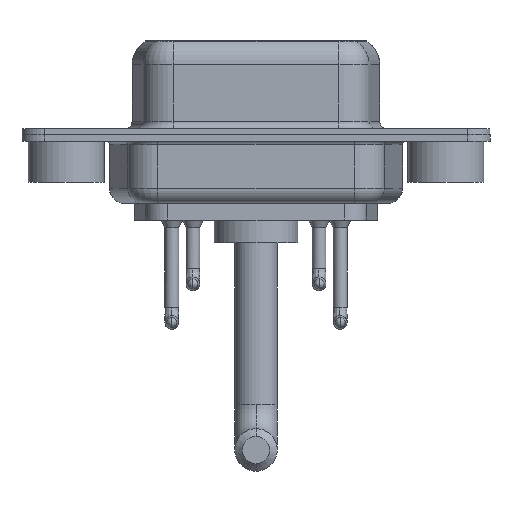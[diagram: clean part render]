
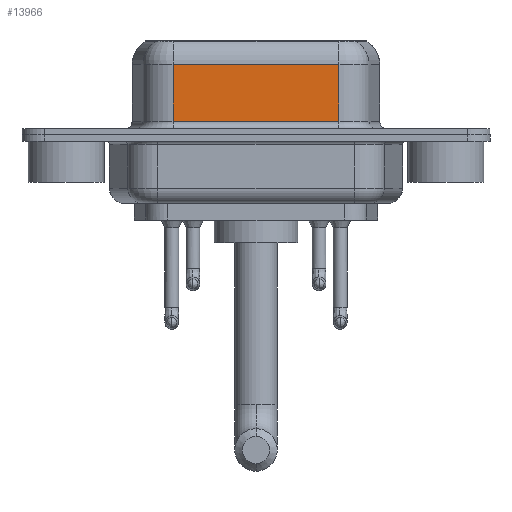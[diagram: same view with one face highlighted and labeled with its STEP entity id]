
A CAD part, front view. The second image highlights one B-rep face of the part: STEP entity #13966.
In plain terms, the highlighted planar face has unit normal (0, -1, 0).
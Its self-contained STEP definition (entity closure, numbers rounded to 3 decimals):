
#657 = LINE ( 'NONE', #3358, #12945 ) ;
#970 = DIRECTION ( 'NONE',  ( -1., 0., 0. ) ) ;
#1508 = VECTOR ( 'NONE', #3778, 1000. ) ;
#1945 = DIRECTION ( 'NONE',  ( 0., 0., -1. ) ) ;
#2116 = ORIENTED_EDGE ( 'NONE', *, *, #2692, .T. ) ;
#2432 = VERTEX_POINT ( 'NONE', #15651 ) ;
#2684 = ORIENTED_EDGE ( 'NONE', *, *, #11382, .T. ) ;
#2692 = EDGE_CURVE ( 'NONE', #11698, #7810, #15080, .T. ) ;
#2936 = LINE ( 'NONE', #4114, #13188 ) ;
#3358 = CARTESIAN_POINT ( 'NONE',  ( 17.962, -3.95, 4.65 ) ) ;
#3413 = ORIENTED_EDGE ( 'NONE', *, *, #6313, .T. ) ;
#3778 = DIRECTION ( 'NONE',  ( 1., 0., 0. ) ) ;
#4114 = CARTESIAN_POINT ( 'NONE',  ( 7.038, -3.95, 6.4 ) ) ;
#5553 = CARTESIAN_POINT ( 'NONE',  ( 7.038, -3.95, 0.9 ) ) ;
#5979 = DIRECTION ( 'NONE',  ( 0., 1., 0. ) ) ;
#6313 = EDGE_CURVE ( 'NONE', #2432, #11698, #2936, .T. ) ;
#7452 = FACE_OUTER_BOUND ( 'NONE', #10672, .T. ) ;
#7810 = VERTEX_POINT ( 'NONE', #12183 ) ;
#9373 = VERTEX_POINT ( 'NONE', #11552 ) ;
#9744 = EDGE_CURVE ( 'NONE', #9373, #7810, #11918, .T. ) ;
#10117 = CARTESIAN_POINT ( 'NONE',  ( 17.962, -3.95, 0.9 ) ) ;
#10529 = CARTESIAN_POINT ( 'NONE',  ( 17.962, -3.95, 6.4 ) ) ;
#10672 = EDGE_LOOP ( 'NONE', ( #15057, #2684, #3413, #2116 ) ) ;
#10815 = VECTOR ( 'NONE', #1945, 1000. ) ;
#11382 = EDGE_CURVE ( 'NONE', #9373, #2432, #657, .T. ) ;
#11552 = CARTESIAN_POINT ( 'NONE',  ( 17.962, -3.95, 4.65 ) ) ;
#11698 = VERTEX_POINT ( 'NONE', #5553 ) ;
#11918 = LINE ( 'NONE', #10529, #10815 ) ;
#12183 = CARTESIAN_POINT ( 'NONE',  ( 17.962, -3.95, 0.9 ) ) ;
#12945 = VECTOR ( 'NONE', #15805, 1000. ) ;
#13188 = VECTOR ( 'NONE', #15166, 1000. ) ;
#13966 = ADVANCED_FACE ( 'NONE', ( #7452 ), #15863, .F. ) ;
#14650 = CARTESIAN_POINT ( 'NONE',  ( 17.962, -3.95, 6.4 ) ) ;
#15057 = ORIENTED_EDGE ( 'NONE', *, *, #9744, .F. ) ;
#15080 = LINE ( 'NONE', #10117, #1508 ) ;
#15123 = AXIS2_PLACEMENT_3D ( 'NONE', #14650, #5979, #970 ) ;
#15166 = DIRECTION ( 'NONE',  ( 0., 0., -1. ) ) ;
#15651 = CARTESIAN_POINT ( 'NONE',  ( 7.038, -3.95, 4.65 ) ) ;
#15805 = DIRECTION ( 'NONE',  ( -1., 0., 0. ) ) ;
#15863 = PLANE ( 'NONE',  #15123 ) ;
